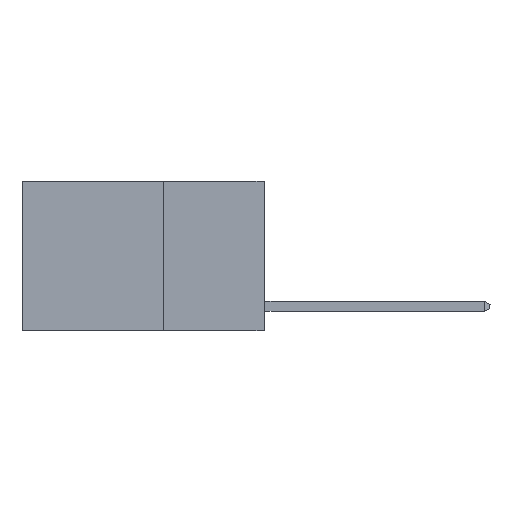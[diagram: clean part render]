
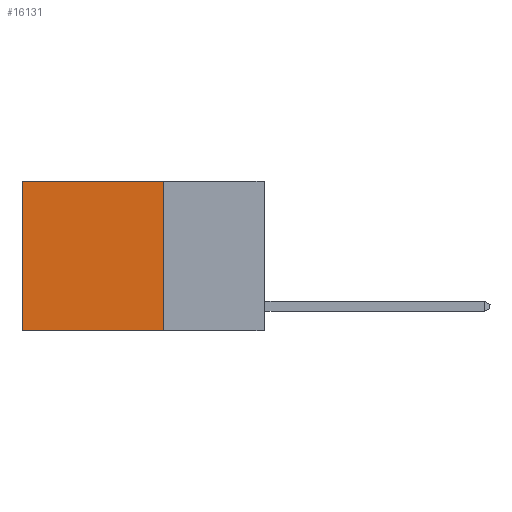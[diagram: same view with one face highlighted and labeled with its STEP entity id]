
A CAD part, left-side view. The second image highlights one B-rep face of the part: STEP entity #16131.
In plain terms, the highlighted planar face has unit normal (-1, 0, 0).
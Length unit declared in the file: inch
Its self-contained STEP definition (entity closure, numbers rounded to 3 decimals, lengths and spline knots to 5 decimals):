
#410 = LINE ( 'NONE', #3444, #18662 ) ;
#567 = CARTESIAN_POINT ( 'NONE',  ( 0.2625, 0.25, 0. ) ) ;
#665 = CARTESIAN_POINT ( 'NONE',  ( 0.2625, 0.25, 0. ) ) ;
#1029 = VECTOR ( 'NONE', #21353, 39.37008 ) ;
#2229 = CARTESIAN_POINT ( 'NONE',  ( 0.2625, 0.6, -0.37 ) ) ;
#2594 = AXIS2_PLACEMENT_3D ( 'NONE', #4581, #16883, #6416 ) ;
#3120 = EDGE_CURVE ( 'NONE', #19505, #7147, #410, .T. ) ;
#3444 = CARTESIAN_POINT ( 'NONE',  ( 0.2625, 0.25, 0. ) ) ;
#3463 = ORIENTED_EDGE ( 'NONE', *, *, #3120, .T. ) ;
#3739 = VERTEX_POINT ( 'NONE', #17284 ) ;
#4581 = CARTESIAN_POINT ( 'NONE',  ( 0.2625, 0.25, 0. ) ) ;
#5810 = EDGE_CURVE ( 'NONE', #3739, #8231, #15074, .T. ) ;
#5890 = LINE ( 'NONE', #11151, #1029 ) ;
#6416 = DIRECTION ( 'NONE',  ( 0., 0., -1. ) ) ;
#7147 = VERTEX_POINT ( 'NONE', #22115 ) ;
#7316 = ORIENTED_EDGE ( 'NONE', *, *, #22016, .F. ) ;
#7891 = LINE ( 'NONE', #567, #20579 ) ;
#7898 = FACE_OUTER_BOUND ( 'NONE', #11667, .T. ) ;
#8231 = VERTEX_POINT ( 'NONE', #2229 ) ;
#8522 = DIRECTION ( 'NONE',  ( 0., 1., 0. ) ) ;
#9975 = ORIENTED_EDGE ( 'NONE', *, *, #11249, .T. ) ;
#11151 = CARTESIAN_POINT ( 'NONE',  ( 0.2625, 0.6, 0. ) ) ;
#11249 = EDGE_CURVE ( 'NONE', #7147, #8231, #5890, .T. ) ;
#11490 = ORIENTED_EDGE ( 'NONE', *, *, #5810, .F. ) ;
#11667 = EDGE_LOOP ( 'NONE', ( #9975, #11490, #7316, #3463 ) ) ;
#11735 = PLANE ( 'NONE',  #2594 ) ;
#14825 = DIRECTION ( 'NONE',  ( 0., 0., -1. ) ) ;
#15074 = LINE ( 'NONE', #18873, #19092 ) ;
#16131 = ADVANCED_FACE ( 'NONE', ( #7898 ), #11735, .F. ) ;
#16883 = DIRECTION ( 'NONE',  ( 1., 0., 0. ) ) ;
#17284 = CARTESIAN_POINT ( 'NONE',  ( 0.2625, 0.25, -0.37 ) ) ;
#18662 = VECTOR ( 'NONE', #19250, 39.37008 ) ;
#18873 = CARTESIAN_POINT ( 'NONE',  ( 0.2625, 0.25, -0.37 ) ) ;
#19092 = VECTOR ( 'NONE', #8522, 39.37008 ) ;
#19250 = DIRECTION ( 'NONE',  ( 0., 1., 0. ) ) ;
#19505 = VERTEX_POINT ( 'NONE', #665 ) ;
#20579 = VECTOR ( 'NONE', #14825, 39.37008 ) ;
#21353 = DIRECTION ( 'NONE',  ( 0., 0., -1. ) ) ;
#22016 = EDGE_CURVE ( 'NONE', #19505, #3739, #7891, .T. ) ;
#22115 = CARTESIAN_POINT ( 'NONE',  ( 0.2625, 0.6, 0. ) ) ;
